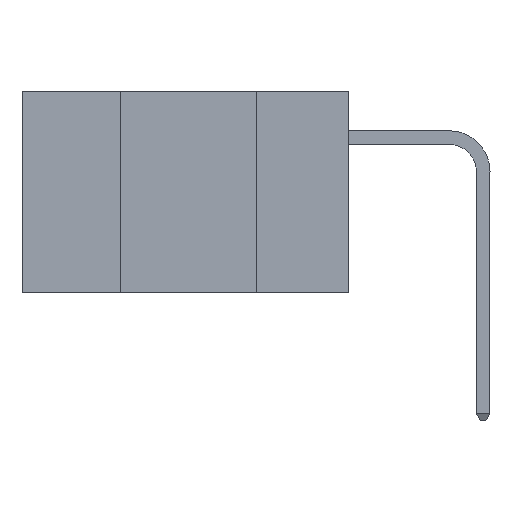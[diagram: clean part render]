
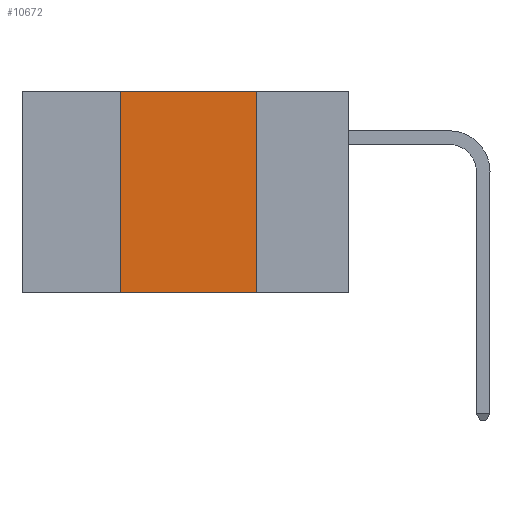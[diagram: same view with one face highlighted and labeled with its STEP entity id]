
A CAD part, left-side view. The second image highlights one B-rep face of the part: STEP entity #10672.
In plain terms, the highlighted planar face has unit normal (-1, 0, 0).
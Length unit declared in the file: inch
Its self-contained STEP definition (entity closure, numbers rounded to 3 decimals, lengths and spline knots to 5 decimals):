
#331 = CARTESIAN_POINT ( 'NONE',  ( 0., 0.17, 0. ) ) ;
#454 = LINE ( 'NONE', #3729, #9655 ) ;
#627 = DIRECTION ( 'NONE',  ( 0., -1., 0. ) ) ;
#688 = VERTEX_POINT ( 'NONE', #2327 ) ;
#1733 = CARTESIAN_POINT ( 'NONE',  ( 0., 0.42, 0. ) ) ;
#1961 = VECTOR ( 'NONE', #627, 39.37008 ) ;
#2327 = CARTESIAN_POINT ( 'NONE',  ( 0., 0.42, 0. ) ) ;
#3063 = ORIENTED_EDGE ( 'NONE', *, *, #11525, .F. ) ;
#3151 = ORIENTED_EDGE ( 'NONE', *, *, #6916, .F. ) ;
#3386 = ORIENTED_EDGE ( 'NONE', *, *, #11635, .F. ) ;
#3537 = ORIENTED_EDGE ( 'NONE', *, *, #11651, .T. ) ;
#3642 = VECTOR ( 'NONE', #3970, 39.37008 ) ;
#3729 = CARTESIAN_POINT ( 'NONE',  ( 0., 0.17, 0. ) ) ;
#3821 = AXIS2_PLACEMENT_3D ( 'NONE', #6949, #4056, #10299 ) ;
#3970 = DIRECTION ( 'NONE',  ( 0., -1., 0. ) ) ;
#4056 = DIRECTION ( 'NONE',  ( 1., 0., 0. ) ) ;
#4589 = LINE ( 'NONE', #6924, #1961 ) ;
#6301 = LINE ( 'NONE', #6873, #3642 ) ;
#6595 = VECTOR ( 'NONE', #8584, 39.37008 ) ;
#6713 = DIRECTION ( 'NONE',  ( 0., 0., -1. ) ) ;
#6873 = CARTESIAN_POINT ( 'NONE',  ( 0., 0.6, -0.37 ) ) ;
#6916 = EDGE_CURVE ( 'NONE', #688, #9395, #4589, .T. ) ;
#6924 = CARTESIAN_POINT ( 'NONE',  ( 0., 0.6, 0. ) ) ;
#6949 = CARTESIAN_POINT ( 'NONE',  ( 0., 0.6, 0. ) ) ;
#6975 = VERTEX_POINT ( 'NONE', #11069 ) ;
#7163 = EDGE_LOOP ( 'NONE', ( #3063, #3151, #3386, #3537 ) ) ;
#7315 = FACE_OUTER_BOUND ( 'NONE', #7163, .T. ) ;
#8584 = DIRECTION ( 'NONE',  ( 0., 0., 1. ) ) ;
#9395 = VERTEX_POINT ( 'NONE', #331 ) ;
#9402 = CARTESIAN_POINT ( 'NONE',  ( 0., 0.42, -0.37 ) ) ;
#9655 = VECTOR ( 'NONE', #6713, 39.37008 ) ;
#10267 = PLANE ( 'NONE',  #3821 ) ;
#10299 = DIRECTION ( 'NONE',  ( 0., 0., -1. ) ) ;
#10672 = ADVANCED_FACE ( 'NONE', ( #7315 ), #10267, .F. ) ;
#10772 = LINE ( 'NONE', #1733, #6595 ) ;
#11069 = CARTESIAN_POINT ( 'NONE',  ( 0., 0.17, -0.37 ) ) ;
#11525 = EDGE_CURVE ( 'NONE', #9395, #6975, #454, .T. ) ;
#11635 = EDGE_CURVE ( 'NONE', #11652, #688, #10772, .T. ) ;
#11651 = EDGE_CURVE ( 'NONE', #11652, #6975, #6301, .T. ) ;
#11652 = VERTEX_POINT ( 'NONE', #9402 ) ;
